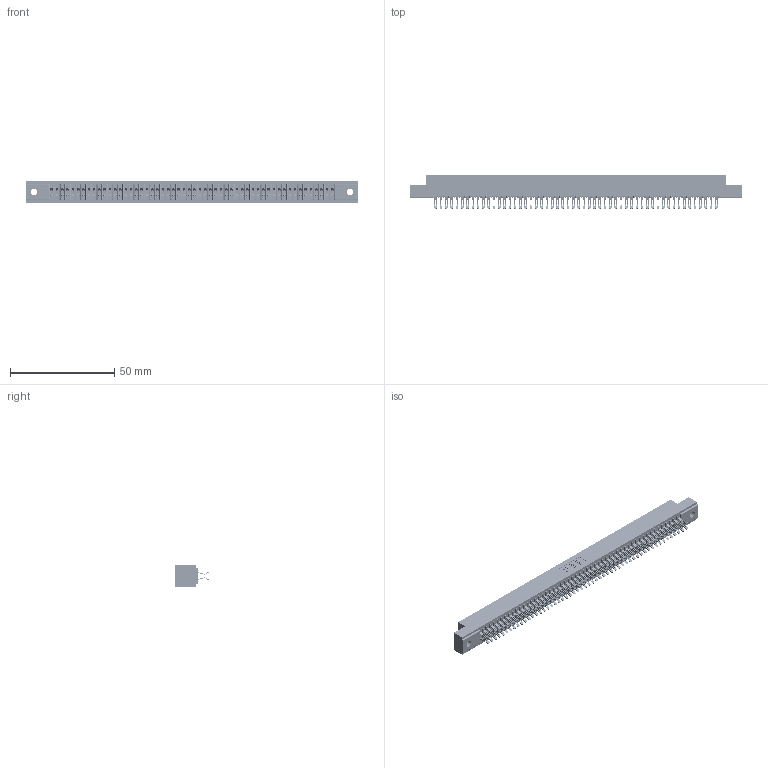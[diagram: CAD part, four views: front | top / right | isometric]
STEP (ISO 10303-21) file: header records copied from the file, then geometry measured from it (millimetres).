
FILE_DESCRIPTION (( 'STEP AP203' ), '1' );
FILE_NAME ('341-108-555-202.STEP', '2018-08-08T12:23:55', ( '' ), ( '' ), 'SwSTEP 2.0', 'SolidWorks 2016', '' );
FILE_SCHEMA (( 'CONFIG_CONTROL_DESIGN' ));
Length unit declared in the file: inch
Products named in the file (3): 341 Part_.128 (3.25) Dia Mounting Holes; 341-292-001_341-292-155; 341-108-555-202
Assembly tree (109 placements, depth 2):
  341-108-555-202
    341 Part_.128 (3.25) Dia Mounting Holes
    341-292-001_341-292-155  x108
Bounding box: 159.38 x 16.31 x 10.16 mm (x, y, z)
Volume: 11877.5 mm3; surface area: 22093.5 mm2
Topology: 109 solids, 109 shells, 8540 faces, 25534 edges, 16622 vertices
Faces by surface type: plane 4604, cylinder 3720, sphere 110, torus 106
Entity records: 64225 total; most frequent: CARTESIAN_POINT 10692, ORIENTED_EDGE 10616, DIRECTION 10358, EDGE_CURVE 5308, LINE 4286, VECTOR 4286, VERTEX_POINT 3354, AXIS2_PLACEMENT_3D 3036
